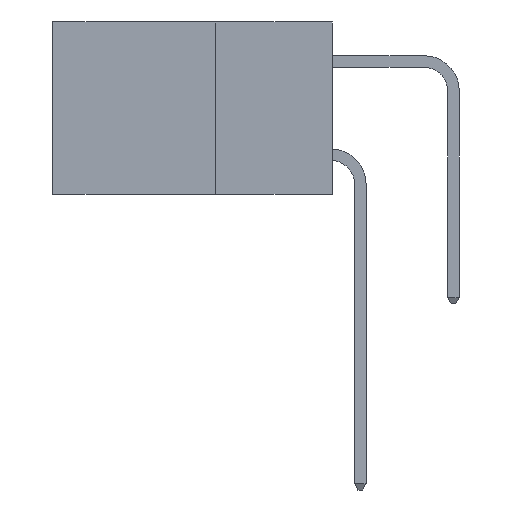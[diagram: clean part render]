
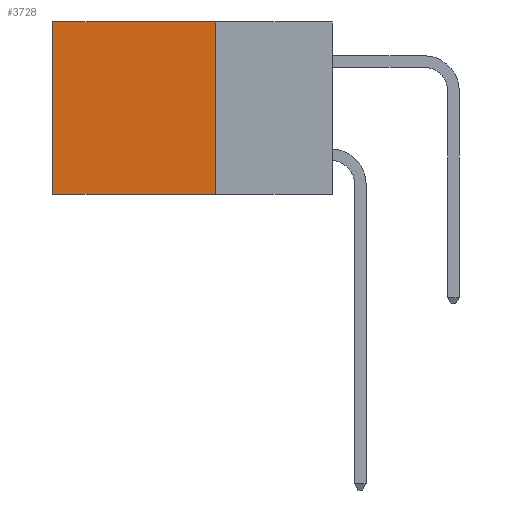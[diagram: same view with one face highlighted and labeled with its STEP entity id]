
A CAD part, left-side view. The second image highlights one B-rep face of the part: STEP entity #3728.
In plain terms, the highlighted planar face has unit normal (-1, 0, 0).
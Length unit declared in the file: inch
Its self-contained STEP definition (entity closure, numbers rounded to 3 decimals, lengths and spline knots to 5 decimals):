
#607 = VECTOR ( 'NONE', #5752, 39.37008 ) ;
#736 = ORIENTED_EDGE ( 'NONE', *, *, #6636, .F. ) ;
#1109 = VERTEX_POINT ( 'NONE', #1195 ) ;
#1160 = ORIENTED_EDGE ( 'NONE', *, *, #7820, .F. ) ;
#1195 = CARTESIAN_POINT ( 'NONE',  ( 0.2615, 0.25, -0.37 ) ) ;
#1225 = DIRECTION ( 'NONE',  ( 0., 0., -1. ) ) ;
#2157 = VECTOR ( 'NONE', #2556, 39.37008 ) ;
#2540 = CARTESIAN_POINT ( 'NONE',  ( 0.2615, 0.25, 0. ) ) ;
#2556 = DIRECTION ( 'NONE',  ( 0., 1., 0. ) ) ;
#2891 = VECTOR ( 'NONE', #1225, 39.37008 ) ;
#2940 = VERTEX_POINT ( 'NONE', #6514 ) ;
#3156 = VECTOR ( 'NONE', #15746, 39.37008 ) ;
#3361 = CARTESIAN_POINT ( 'NONE',  ( 0.2615, 0.6, 0. ) ) ;
#3728 = ADVANCED_FACE ( 'NONE', ( #8948 ), #5504, .F. ) ;
#3845 = VERTEX_POINT ( 'NONE', #3361 ) ;
#3974 = LINE ( 'NONE', #15882, #3156 ) ;
#5085 = DIRECTION ( 'NONE',  ( 0., 0., -1. ) ) ;
#5107 = DIRECTION ( 'NONE',  ( 1., 0., 0. ) ) ;
#5139 = CARTESIAN_POINT ( 'NONE',  ( 0.2615, 0.25, -0.37 ) ) ;
#5290 = CARTESIAN_POINT ( 'NONE',  ( 0.2615, 0.6, -0.37 ) ) ;
#5504 = PLANE ( 'NONE',  #7533 ) ;
#5661 = LINE ( 'NONE', #2540, #2157 ) ;
#5694 = CARTESIAN_POINT ( 'NONE',  ( 0.2615, 0.25, -0.37 ) ) ;
#5752 = DIRECTION ( 'NONE',  ( 0., 0., -1. ) ) ;
#6514 = CARTESIAN_POINT ( 'NONE',  ( 0.2615, 0.25, 0. ) ) ;
#6636 = EDGE_CURVE ( 'NONE', #1109, #10620, #3974, .T. ) ;
#7288 = ORIENTED_EDGE ( 'NONE', *, *, #16004, .T. ) ;
#7533 = AXIS2_PLACEMENT_3D ( 'NONE', #5139, #5107, #5085 ) ;
#7820 = EDGE_CURVE ( 'NONE', #2940, #1109, #14027, .T. ) ;
#8133 = ORIENTED_EDGE ( 'NONE', *, *, #11003, .T. ) ;
#8948 = FACE_OUTER_BOUND ( 'NONE', #11893, .T. ) ;
#10394 = CARTESIAN_POINT ( 'NONE',  ( 0.2615, 0.6, -0.37 ) ) ;
#10620 = VERTEX_POINT ( 'NONE', #5290 ) ;
#11003 = EDGE_CURVE ( 'NONE', #2940, #3845, #5661, .T. ) ;
#11893 = EDGE_LOOP ( 'NONE', ( #7288, #736, #1160, #8133 ) ) ;
#12879 = LINE ( 'NONE', #10394, #2891 ) ;
#14027 = LINE ( 'NONE', #5694, #607 ) ;
#15746 = DIRECTION ( 'NONE',  ( 0., 1., 0. ) ) ;
#15882 = CARTESIAN_POINT ( 'NONE',  ( 0.2615, 0.25, -0.37 ) ) ;
#16004 = EDGE_CURVE ( 'NONE', #3845, #10620, #12879, .T. ) ;
